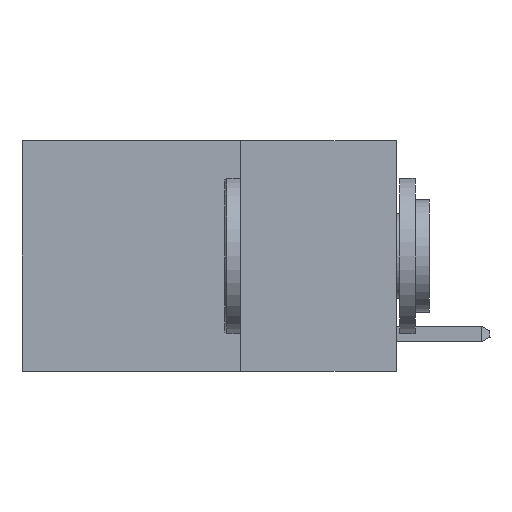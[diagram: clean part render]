
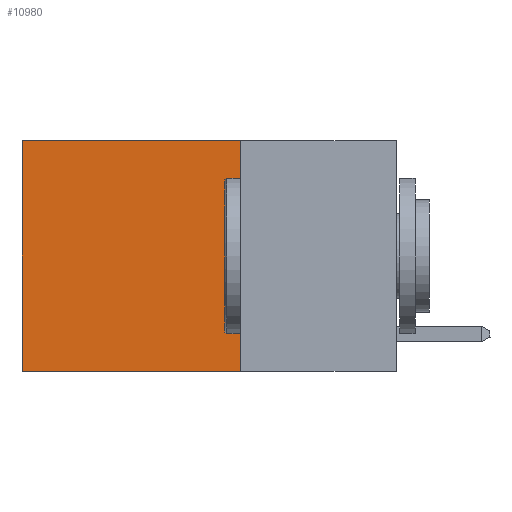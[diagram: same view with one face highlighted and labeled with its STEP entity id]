
A CAD part, left-side view. The second image highlights one B-rep face of the part: STEP entity #10980.
In plain terms, the highlighted planar face has unit normal (-1, 0, 0).
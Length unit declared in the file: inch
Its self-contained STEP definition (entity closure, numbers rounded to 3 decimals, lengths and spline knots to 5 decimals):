
#18 = DIRECTION ( 'NONE',  ( 0., 0., -1. ) ) ;
#21 = EDGE_LOOP ( 'NONE', ( #3349, #9035, #7846, #8174 ) ) ;
#267 = VERTEX_POINT ( 'NONE', #11223 ) ;
#442 = CARTESIAN_POINT ( 'NONE',  ( 0.2625, 0.25, 0. ) ) ;
#594 = VERTEX_POINT ( 'NONE', #2647 ) ;
#754 = EDGE_CURVE ( 'NONE', #594, #2503, #8969, .T. ) ;
#974 = LINE ( 'NONE', #11387, #8547 ) ;
#1360 = VERTEX_POINT ( 'NONE', #12028 ) ;
#2017 = PLANE ( 'NONE',  #6101 ) ;
#2503 = VERTEX_POINT ( 'NONE', #4312 ) ;
#2647 = CARTESIAN_POINT ( 'NONE',  ( 0.2625, 0.25, 0. ) ) ;
#3097 = DIRECTION ( 'NONE',  ( 0., 0., -1. ) ) ;
#3349 = ORIENTED_EDGE ( 'NONE', *, *, #12878, .T. ) ;
#3598 = VECTOR ( 'NONE', #7815, 39.37008 ) ;
#4312 = CARTESIAN_POINT ( 'NONE',  ( 0.2625, 0.25, -0.37 ) ) ;
#5368 = DIRECTION ( 'NONE',  ( 0., 1., 0. ) ) ;
#6101 = AXIS2_PLACEMENT_3D ( 'NONE', #6181, #9196, #3097 ) ;
#6181 = CARTESIAN_POINT ( 'NONE',  ( 0.2625, 0.25, 0. ) ) ;
#6315 = VECTOR ( 'NONE', #13109, 39.37008 ) ;
#6362 = LINE ( 'NONE', #8823, #3598 ) ;
#7815 = DIRECTION ( 'NONE',  ( 0., 1., 0. ) ) ;
#7846 = ORIENTED_EDGE ( 'NONE', *, *, #754, .F. ) ;
#8174 = ORIENTED_EDGE ( 'NONE', *, *, #8868, .T. ) ;
#8330 = VECTOR ( 'NONE', #18, 39.37008 ) ;
#8547 = VECTOR ( 'NONE', #5368, 39.37008 ) ;
#8656 = LINE ( 'NONE', #10318, #8330 ) ;
#8682 = EDGE_CURVE ( 'NONE', #2503, #1360, #974, .T. ) ;
#8823 = CARTESIAN_POINT ( 'NONE',  ( 0.2625, 0.25, 0. ) ) ;
#8868 = EDGE_CURVE ( 'NONE', #594, #267, #6362, .T. ) ;
#8969 = LINE ( 'NONE', #442, #6315 ) ;
#9035 = ORIENTED_EDGE ( 'NONE', *, *, #8682, .F. ) ;
#9196 = DIRECTION ( 'NONE',  ( 1., 0., 0. ) ) ;
#10318 = CARTESIAN_POINT ( 'NONE',  ( 0.2625, 0.6, 0. ) ) ;
#10980 = ADVANCED_FACE ( 'NONE', ( #12200 ), #2017, .F. ) ;
#11223 = CARTESIAN_POINT ( 'NONE',  ( 0.2625, 0.6, 0. ) ) ;
#11387 = CARTESIAN_POINT ( 'NONE',  ( 0.2625, 0.25, -0.37 ) ) ;
#12028 = CARTESIAN_POINT ( 'NONE',  ( 0.2625, 0.6, -0.37 ) ) ;
#12200 = FACE_OUTER_BOUND ( 'NONE', #21, .T. ) ;
#12878 = EDGE_CURVE ( 'NONE', #267, #1360, #8656, .T. ) ;
#13109 = DIRECTION ( 'NONE',  ( 0., 0., -1. ) ) ;
